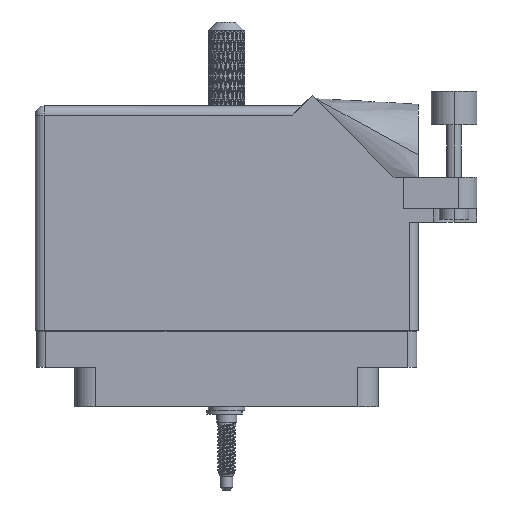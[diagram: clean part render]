
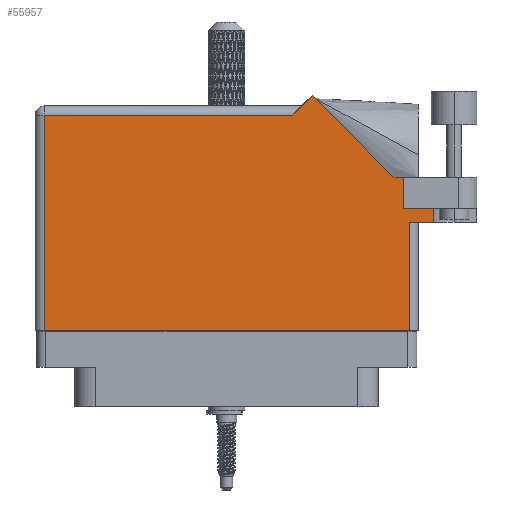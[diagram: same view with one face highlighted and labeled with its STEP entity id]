
A CAD part, front view. The second image highlights one B-rep face of the part: STEP entity #55957.
In plain terms, the highlighted face is planar.
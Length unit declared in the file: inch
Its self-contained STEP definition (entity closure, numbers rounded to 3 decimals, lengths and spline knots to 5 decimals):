
#435 = CARTESIAN_POINT ( 'NONE',  ( 0.451, 1.368, 0.455 ) ) ;
#1619 = CARTESIAN_POINT ( 'NONE',  ( 1.244, 0.637, 0.455 ) ) ;
#1914 = VECTOR ( 'NONE', #55115, 39.37008 ) ;
#1970 = CARTESIAN_POINT ( 'NONE',  ( -1.306, -0.1, 0.455 ) ) ;
#3484 = DIRECTION ( 'NONE',  ( -0.707, 0.707, 0. ) ) ;
#3710 = VERTEX_POINT ( 'NONE', #76241 ) ;
#4270 = EDGE_CURVE ( 'NONE', #77512, #54624, #20984, .T. ) ;
#5516 = CARTESIAN_POINT ( 'NONE',  ( 1.206, 0.731, 0.455 ) ) ;
#11264 = VECTOR ( 'NONE', #109834, 39.37008 ) ;
#12962 = CARTESIAN_POINT ( 'NONE',  ( 1.14042, 0.944, 0.455 ) ) ;
#13360 = LINE ( 'NONE', #87749, #101649 ) ;
#15601 = PLANE ( 'NONE',  #28340 ) ;
#15797 = CARTESIAN_POINT ( 'NONE',  ( 0.58371, 1.50071, 0.455 ) ) ;
#18420 = DIRECTION ( 'NONE',  ( -1., 0., 0. ) ) ;
#20984 = LINE ( 'NONE', #90385, #114996 ) ;
#23070 = CARTESIAN_POINT ( 'NONE',  ( -1.244, 1.368, 0.455 ) ) ;
#23416 = DIRECTION ( 'NONE',  ( 1., 0., 0. ) ) ;
#23714 = CARTESIAN_POINT ( 'NONE',  ( 1.206, 0.944, 0.455 ) ) ;
#24749 = CARTESIAN_POINT ( 'NONE',  ( -1.306, 1.43, 0.455 ) ) ;
#25486 = LINE ( 'NONE', #1970, #113794 ) ;
#26301 = DIRECTION ( 'NONE',  ( 0., 1., 0. ) ) ;
#26800 = EDGE_CURVE ( 'NONE', #85340, #77512, #100790, .T. ) ;
#26889 = VERTEX_POINT ( 'NONE', #88776 ) ;
#27611 = VERTEX_POINT ( 'NONE', #83935 ) ;
#28340 = AXIS2_PLACEMENT_3D ( 'NONE', #24749, #88615, #18420 ) ;
#32483 = DIRECTION ( 'NONE',  ( -0.707, -0.707, 0. ) ) ;
#32529 = EDGE_CURVE ( 'NONE', #26889, #55099, #73019, .T. ) ;
#32710 = VERTEX_POINT ( 'NONE', #107738 ) ;
#36058 = CARTESIAN_POINT ( 'NONE',  ( -1.244, -0.1, 0.455 ) ) ;
#36593 = VECTOR ( 'NONE', #23416, 39.37008 ) ;
#39148 = LINE ( 'NONE', #1619, #50465 ) ;
#41153 = LINE ( 'NONE', #110623, #11264 ) ;
#44266 = VERTEX_POINT ( 'NONE', #50038 ) ;
#45529 = FACE_OUTER_BOUND ( 'NONE', #116731, .T. ) ;
#50038 = CARTESIAN_POINT ( 'NONE',  ( 1.4075, 0.637, 0.455 ) ) ;
#50465 = VECTOR ( 'NONE', #91656, 39.37008 ) ;
#51528 = ORIENTED_EDGE ( 'NONE', *, *, #83207, .T. ) ;
#52246 = EDGE_CURVE ( 'NONE', #60989, #3710, #25486, .T. ) ;
#53882 = ORIENTED_EDGE ( 'NONE', *, *, #101706, .F. ) ;
#54624 = VERTEX_POINT ( 'NONE', #23070 ) ;
#55099 = VERTEX_POINT ( 'NONE', #23714 ) ;
#55115 = DIRECTION ( 'NONE',  ( 0., -1., 0. ) ) ;
#55957 = ADVANCED_FACE ( 'NONE', ( #45529 ), #15601, .F. ) ;
#57747 = EDGE_CURVE ( 'NONE', #26889, #32710, #72255, .T. ) ;
#59623 = ORIENTED_EDGE ( 'NONE', *, *, #77500, .T. ) ;
#60989 = VERTEX_POINT ( 'NONE', #70418 ) ;
#67544 = ORIENTED_EDGE ( 'NONE', *, *, #4270, .T. ) ;
#69437 = EDGE_CURVE ( 'NONE', #54624, #60989, #97374, .T. ) ;
#69587 = DIRECTION ( 'NONE',  ( 1., 0., 0. ) ) ;
#70418 = CARTESIAN_POINT ( 'NONE',  ( -1.244, -0.1, 0.455 ) ) ;
#70829 = VECTOR ( 'NONE', #106362, 39.37008 ) ;
#72255 = LINE ( 'NONE', #5516, #36593 ) ;
#72402 = LINE ( 'NONE', #12962, #81106 ) ;
#73019 = LINE ( 'NONE', #97607, #91569 ) ;
#74247 = EDGE_CURVE ( 'NONE', #55099, #99335, #109318, .T. ) ;
#76241 = CARTESIAN_POINT ( 'NONE',  ( 1.244, -0.1, 0.455 ) ) ;
#77500 = EDGE_CURVE ( 'NONE', #3710, #27611, #39148, .T. ) ;
#77512 = VERTEX_POINT ( 'NONE', #435 ) ;
#78628 = EDGE_CURVE ( 'NONE', #27611, #44266, #13360, .T. ) ;
#79324 = ORIENTED_EDGE ( 'NONE', *, *, #69437, .T. ) ;
#79897 = ORIENTED_EDGE ( 'NONE', *, *, #57747, .F. ) ;
#81083 = ORIENTED_EDGE ( 'NONE', *, *, #78628, .T. ) ;
#81106 = VECTOR ( 'NONE', #3484, 39.37008 ) ;
#83207 = EDGE_CURVE ( 'NONE', #99335, #85340, #72402, .T. ) ;
#83935 = CARTESIAN_POINT ( 'NONE',  ( 1.244, 0.637, 0.455 ) ) ;
#85340 = VERTEX_POINT ( 'NONE', #15797 ) ;
#87749 = CARTESIAN_POINT ( 'NONE',  ( 1.306, 0.637, 0.455 ) ) ;
#88615 = DIRECTION ( 'NONE',  ( 0., 0., -1. ) ) ;
#88776 = CARTESIAN_POINT ( 'NONE',  ( 1.206, 0.731, 0.455 ) ) ;
#90166 = ORIENTED_EDGE ( 'NONE', *, *, #26800, .T. ) ;
#90385 = CARTESIAN_POINT ( 'NONE',  ( -1.306, 1.368, 0.455 ) ) ;
#91569 = VECTOR ( 'NONE', #26301, 39.37008 ) ;
#91656 = DIRECTION ( 'NONE',  ( 0., 1., 0. ) ) ;
#97071 = CARTESIAN_POINT ( 'NONE',  ( 0.513, 1.43, 0.455 ) ) ;
#97312 = CARTESIAN_POINT ( 'NONE',  ( 1.706, 0.944, 0.455 ) ) ;
#97374 = LINE ( 'NONE', #36058, #1914 ) ;
#97607 = CARTESIAN_POINT ( 'NONE',  ( 1.206, 0.731, 0.455 ) ) ;
#98899 = ORIENTED_EDGE ( 'NONE', *, *, #74247, .T. ) ;
#99335 = VERTEX_POINT ( 'NONE', #109655 ) ;
#99471 = VECTOR ( 'NONE', #32483, 39.37008 ) ;
#100790 = LINE ( 'NONE', #97071, #99471 ) ;
#101409 = DIRECTION ( 'NONE',  ( 1., 0., 0. ) ) ;
#101649 = VECTOR ( 'NONE', #69587, 39.37008 ) ;
#101706 = EDGE_CURVE ( 'NONE', #32710, #44266, #41153, .T. ) ;
#101991 = ORIENTED_EDGE ( 'NONE', *, *, #52246, .T. ) ;
#106362 = DIRECTION ( 'NONE',  ( -1., 0., 0. ) ) ;
#107689 = ORIENTED_EDGE ( 'NONE', *, *, #32529, .T. ) ;
#107738 = CARTESIAN_POINT ( 'NONE',  ( 1.4075, 0.731, 0.455 ) ) ;
#109318 = LINE ( 'NONE', #97312, #70829 ) ;
#109348 = DIRECTION ( 'NONE',  ( -1., 0., 0. ) ) ;
#109655 = CARTESIAN_POINT ( 'NONE',  ( 1.14042, 0.944, 0.455 ) ) ;
#109834 = DIRECTION ( 'NONE',  ( 0., -1., 0. ) ) ;
#110623 = CARTESIAN_POINT ( 'NONE',  ( 1.4075, 1.06177, 0.455 ) ) ;
#113794 = VECTOR ( 'NONE', #101409, 39.37008 ) ;
#114996 = VECTOR ( 'NONE', #109348, 39.37008 ) ;
#116731 = EDGE_LOOP ( 'NONE', ( #101991, #59623, #81083, #53882, #79897, #107689, #98899, #51528, #90166, #67544, #79324 ) ) ;
